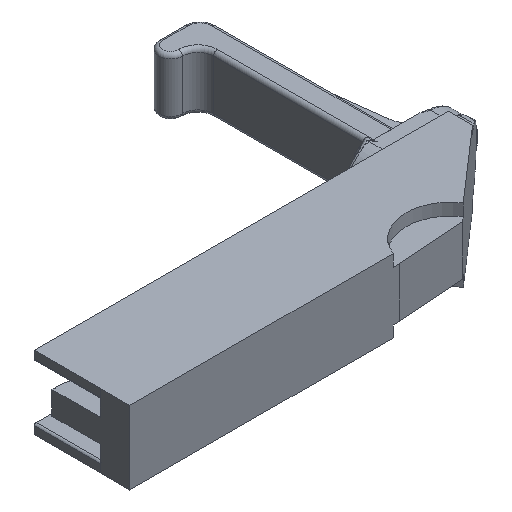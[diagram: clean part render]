
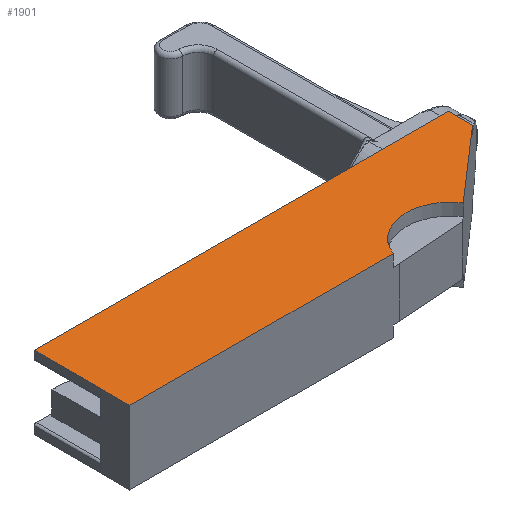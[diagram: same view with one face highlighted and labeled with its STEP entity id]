
A CAD part, isometric view. The second image highlights one B-rep face of the part: STEP entity #1901.
In plain terms, the highlighted planar face has unit normal (0, 0, 1).
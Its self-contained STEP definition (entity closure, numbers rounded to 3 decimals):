
#42=PLANE('',#2049);
#147=FACE_OUTER_BOUND('',#256,.T.);
#256=EDGE_LOOP('',(#1493,#1494,#1495,#1496,#1497,#1498,#1499,#1500));
#346=LINE('',#10491,#490);
#361=LINE('',#10528,#505);
#374=LINE('',#10566,#518);
#399=LINE('',#10695,#543);
#400=LINE('',#10699,#544);
#401=LINE('',#10700,#545);
#402=LINE('',#10701,#546);
#490=VECTOR('',#2253,10.);
#505=VECTOR('',#2284,10.);
#518=VECTOR('',#2329,10.);
#543=VECTOR('',#2374,10.);
#544=VECTOR('',#2377,10.);
#545=VECTOR('',#2378,10.);
#546=VECTOR('',#2379,10.);
#706=CIRCLE('',#2050,5.718);
#815=VERTEX_POINT('',#10488);
#816=VERTEX_POINT('',#10490);
#830=VERTEX_POINT('',#10526);
#838=VERTEX_POINT('',#10563);
#839=VERTEX_POINT('',#10565);
#857=VERTEX_POINT('',#10694);
#858=VERTEX_POINT('',#10696);
#859=VERTEX_POINT('',#10698);
#1023=EDGE_CURVE('',#816,#815,#346,.T.);
#1043=EDGE_CURVE('',#815,#830,#361,.T.);
#1061=EDGE_CURVE('',#839,#838,#374,.T.);
#1096=EDGE_CURVE('',#830,#857,#399,.T.);
#1097=EDGE_CURVE('',#857,#858,#706,.T.);
#1098=EDGE_CURVE('',#858,#859,#400,.T.);
#1099=EDGE_CURVE('',#859,#839,#401,.T.);
#1100=EDGE_CURVE('',#838,#816,#402,.T.);
#1493=ORIENTED_EDGE('',*,*,#1096,.T.);
#1494=ORIENTED_EDGE('',*,*,#1097,.T.);
#1495=ORIENTED_EDGE('',*,*,#1098,.T.);
#1496=ORIENTED_EDGE('',*,*,#1099,.T.);
#1497=ORIENTED_EDGE('',*,*,#1061,.T.);
#1498=ORIENTED_EDGE('',*,*,#1100,.T.);
#1499=ORIENTED_EDGE('',*,*,#1023,.T.);
#1500=ORIENTED_EDGE('',*,*,#1043,.T.);
#1901=ADVANCED_FACE('',(#147),#42,.T.);
#2049=AXIS2_PLACEMENT_3D('',#10693,#2372,#2373);
#2050=AXIS2_PLACEMENT_3D('',#10697,#2375,#2376);
#2253=DIRECTION('',(-1.,0.,0.));
#2284=DIRECTION('',(0.,-1.,0.));
#2329=DIRECTION('',(-1.,0.,0.));
#2372=DIRECTION('center_axis',(0.,0.,1.));
#2373=DIRECTION('ref_axis',(1.,0.,0.));
#2374=DIRECTION('',(1.,0.,0.));
#2375=DIRECTION('center_axis',(0.,0.,-1.));
#2376=DIRECTION('ref_axis',(-0.997,-0.071,0.));
#2377=DIRECTION('',(0.754,0.657,0.));
#2378=DIRECTION('',(0.,1.,0.));
#2379=DIRECTION('',(0.,-1.,0.));
#10488=CARTESIAN_POINT('',(30.4,-8.476,4.683));
#10490=CARTESIAN_POINT('',(30.414,-8.476,4.683));
#10491=CARTESIAN_POINT('',(30.414,-8.476,4.683));
#10526=CARTESIAN_POINT('',(30.4,-12.259,4.683));
#10528=CARTESIAN_POINT('',(30.4,-8.476,4.683));
#10563=CARTESIAN_POINT('',(30.414,0.,4.683));
#10565=CARTESIAN_POINT('',(83.427,0.,4.683));
#10566=CARTESIAN_POINT('',(76.,0.,4.683));
#10693=CARTESIAN_POINT('Origin',(56.867,-5.476,4.683));
#10694=CARTESIAN_POINT('',(64.125,-12.259,4.683));
#10695=CARTESIAN_POINT('',(30.4,-12.259,4.683));
#10696=CARTESIAN_POINT('',(74.23,-11.133,4.683));
#10697=CARTESIAN_POINT('Origin',(69.467,-14.298,4.683));
#10698=CARTESIAN_POINT('',(83.427,-3.115,4.683));
#10699=CARTESIAN_POINT('',(73.648,-11.641,4.683));
#10700=CARTESIAN_POINT('',(83.427,-3.115,4.683));
#10701=CARTESIAN_POINT('',(30.414,0.,4.683));
